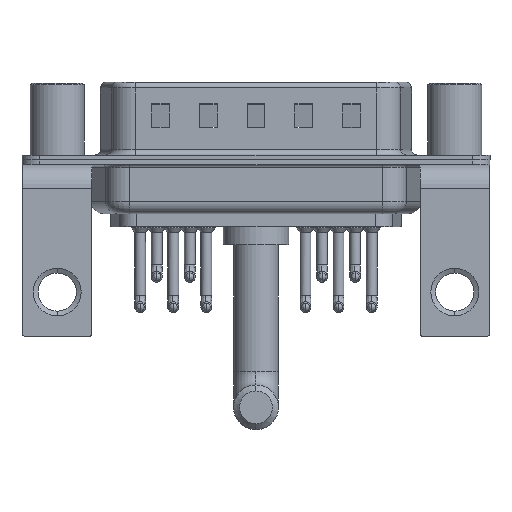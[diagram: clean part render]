
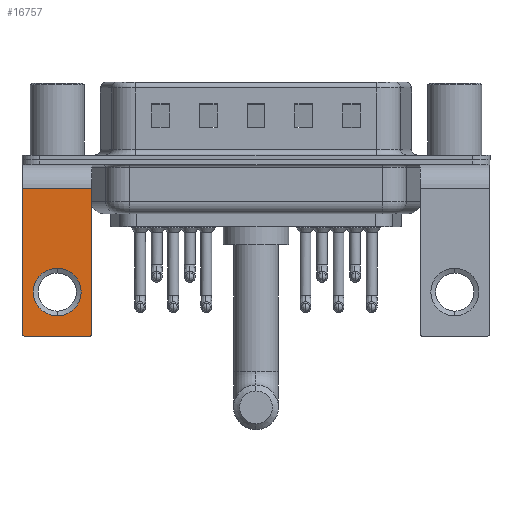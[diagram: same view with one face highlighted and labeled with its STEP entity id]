
A CAD part, front view. The second image highlights one B-rep face of the part: STEP entity #16757.
In plain terms, the highlighted planar face has unit normal (0, -1, 0).
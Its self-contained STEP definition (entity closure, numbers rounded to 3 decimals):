
#1305 = DIRECTION ( 'NONE',  ( 0., 0., 1. ) ) ;
#1595 = CIRCLE ( 'NONE', #20908, 0.25 ) ;
#1716 = CARTESIAN_POINT ( 'NONE',  ( 0., -6.25, -9.07 ) ) ;
#1814 = LINE ( 'NONE', #21085, #13589 ) ;
#1923 = CARTESIAN_POINT ( 'NONE',  ( 2.65, -6.25, -14.8 ) ) ;
#1965 = CARTESIAN_POINT ( 'NONE',  ( 2.9, -6.25, -2.4 ) ) ;
#2593 = PLANE ( 'NONE',  #8208 ) ;
#2622 = EDGE_CURVE ( 'NONE', #20977, #21391, #14157, .T. ) ;
#3724 = DIRECTION ( 'NONE',  ( 0., 1., 0. ) ) ;
#4952 = CIRCLE ( 'NONE', #5364, 2. ) ;
#5364 = AXIS2_PLACEMENT_3D ( 'NONE', #19347, #3724, #23122 ) ;
#5850 = ORIENTED_EDGE ( 'NONE', *, *, #15297, .T. ) ;
#5879 = DIRECTION ( 'NONE',  ( 0., 0., -1. ) ) ;
#6141 = FACE_OUTER_BOUND ( 'NONE', #7146, .T. ) ;
#7146 = EDGE_LOOP ( 'NONE', ( #17116, #16612, #15483, #8745, #22501, #15420 ) ) ;
#7339 = EDGE_CURVE ( 'NONE', #24257, #12860, #13282, .T. ) ;
#7397 = VERTEX_POINT ( 'NONE', #11649 ) ;
#7413 = ORIENTED_EDGE ( 'NONE', *, *, #12431, .T. ) ;
#8028 = CARTESIAN_POINT ( 'NONE',  ( 2.9, -6.25, -2.4 ) ) ;
#8208 = AXIS2_PLACEMENT_3D ( 'NONE', #8028, #12037, #19976 ) ;
#8349 = EDGE_LOOP ( 'NONE', ( #5850, #7413 ) ) ;
#8685 = CARTESIAN_POINT ( 'NONE',  ( -2.9, -6.25, -14.55 ) ) ;
#8745 = ORIENTED_EDGE ( 'NONE', *, *, #24082, .T. ) ;
#9441 = CARTESIAN_POINT ( 'NONE',  ( 0., -6.25, -13.07 ) ) ;
#9486 = DIRECTION ( 'NONE',  ( -1., 0., 0. ) ) ;
#9488 = VECTOR ( 'NONE', #5879, 1000. ) ;
#10218 = DIRECTION ( 'NONE',  ( 0., 0., 1. ) ) ;
#10899 = DIRECTION ( 'NONE',  ( 0., 1., 0. ) ) ;
#11649 = CARTESIAN_POINT ( 'NONE',  ( -2.9, -6.25, -2.4 ) ) ;
#12037 = DIRECTION ( 'NONE',  ( 0., 1., 0. ) ) ;
#12431 = EDGE_CURVE ( 'NONE', #15017, #19384, #20490, .T. ) ;
#12587 = VECTOR ( 'NONE', #21064, 1000. ) ;
#12860 = VERTEX_POINT ( 'NONE', #22708 ) ;
#12894 = CARTESIAN_POINT ( 'NONE',  ( -2.65, -6.25, -14.8 ) ) ;
#13244 = CARTESIAN_POINT ( 'NONE',  ( -2.9, -6.25, -2.4 ) ) ;
#13282 = LINE ( 'NONE', #1965, #9488 ) ;
#13363 = LINE ( 'NONE', #13244, #12587 ) ;
#13380 = CARTESIAN_POINT ( 'NONE',  ( 2.9, -6.25, -14.8 ) ) ;
#13589 = VECTOR ( 'NONE', #9486, 1000. ) ;
#14157 = CIRCLE ( 'NONE', #16967, 0.25 ) ;
#15017 = VERTEX_POINT ( 'NONE', #1716 ) ;
#15297 = EDGE_CURVE ( 'NONE', #19384, #15017, #4952, .T. ) ;
#15420 = ORIENTED_EDGE ( 'NONE', *, *, #22817, .T. ) ;
#15483 = ORIENTED_EDGE ( 'NONE', *, *, #15665, .F. ) ;
#15665 = EDGE_CURVE ( 'NONE', #19029, #21391, #18946, .T. ) ;
#15873 = CARTESIAN_POINT ( 'NONE',  ( -2.65, -6.25, -14.55 ) ) ;
#16612 = ORIENTED_EDGE ( 'NONE', *, *, #2622, .T. ) ;
#16632 = DIRECTION ( 'NONE',  ( 0., -1., 0. ) ) ;
#16757 = ADVANCED_FACE ( 'NONE', ( #17696, #6141 ), #2593, .F. ) ;
#16967 = AXIS2_PLACEMENT_3D ( 'NONE', #15873, #23824, #10218 ) ;
#17116 = ORIENTED_EDGE ( 'NONE', *, *, #17627, .T. ) ;
#17627 = EDGE_CURVE ( 'NONE', #7397, #20977, #13363, .T. ) ;
#17696 = FACE_BOUND ( 'NONE', #8349, .T. ) ;
#18549 = CARTESIAN_POINT ( 'NONE',  ( 2.65, -6.25, -14.55 ) ) ;
#18581 = DIRECTION ( 'NONE',  ( 0., 0., 1. ) ) ;
#18946 = LINE ( 'NONE', #13380, #22656 ) ;
#19029 = VERTEX_POINT ( 'NONE', #1923 ) ;
#19347 = CARTESIAN_POINT ( 'NONE',  ( 0., -6.25, -11.07 ) ) ;
#19384 = VERTEX_POINT ( 'NONE', #9441 ) ;
#19706 = AXIS2_PLACEMENT_3D ( 'NONE', #24245, #10899, #18581 ) ;
#19976 = DIRECTION ( 'NONE',  ( 0., 0., 1. ) ) ;
#20490 = CIRCLE ( 'NONE', #19706, 2. ) ;
#20908 = AXIS2_PLACEMENT_3D ( 'NONE', #18549, #16632, #1305 ) ;
#20977 = VERTEX_POINT ( 'NONE', #8685 ) ;
#21059 = CARTESIAN_POINT ( 'NONE',  ( 2.9, -6.25, -2.4 ) ) ;
#21064 = DIRECTION ( 'NONE',  ( 0., 0., -1. ) ) ;
#21085 = CARTESIAN_POINT ( 'NONE',  ( 2.9, -6.25, -2.4 ) ) ;
#21391 = VERTEX_POINT ( 'NONE', #12894 ) ;
#22501 = ORIENTED_EDGE ( 'NONE', *, *, #7339, .F. ) ;
#22656 = VECTOR ( 'NONE', #24484, 1000. ) ;
#22708 = CARTESIAN_POINT ( 'NONE',  ( 2.9, -6.25, -14.55 ) ) ;
#22817 = EDGE_CURVE ( 'NONE', #24257, #7397, #1814, .T. ) ;
#23122 = DIRECTION ( 'NONE',  ( 0., 0., 1. ) ) ;
#23824 = DIRECTION ( 'NONE',  ( 0., -1., 0. ) ) ;
#24082 = EDGE_CURVE ( 'NONE', #19029, #12860, #1595, .T. ) ;
#24245 = CARTESIAN_POINT ( 'NONE',  ( 0., -6.25, -11.07 ) ) ;
#24257 = VERTEX_POINT ( 'NONE', #21059 ) ;
#24484 = DIRECTION ( 'NONE',  ( -1., 0., 0. ) ) ;
